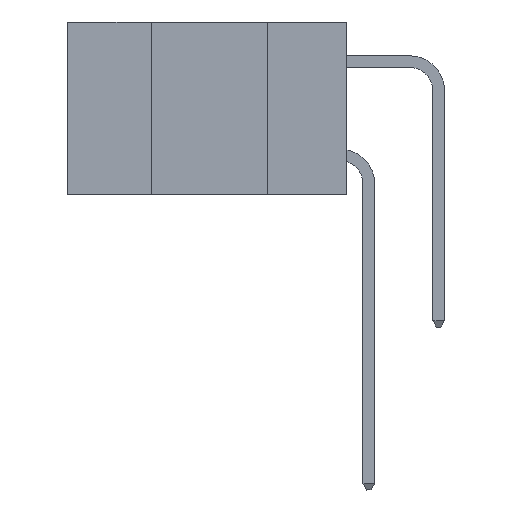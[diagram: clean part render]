
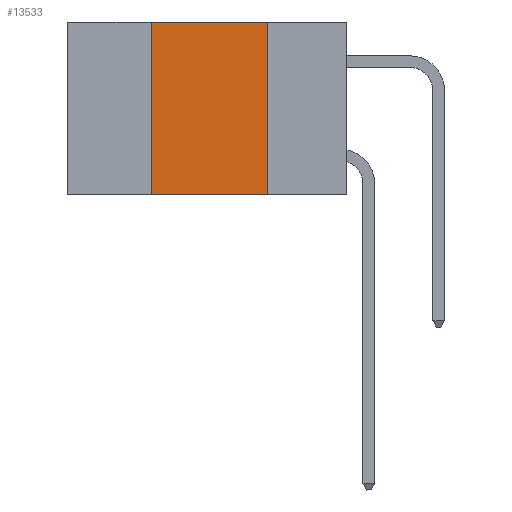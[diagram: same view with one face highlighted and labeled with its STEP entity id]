
A CAD part, left-side view. The second image highlights one B-rep face of the part: STEP entity #13533.
In plain terms, the highlighted planar face has unit normal (-1, 0, 0).
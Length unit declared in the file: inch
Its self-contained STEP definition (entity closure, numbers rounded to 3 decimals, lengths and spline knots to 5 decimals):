
#81 = CARTESIAN_POINT ( 'NONE',  ( 0., 0.42, 0. ) ) ;
#253 = CARTESIAN_POINT ( 'NONE',  ( 0., 0.42, 0. ) ) ;
#668 = VECTOR ( 'NONE', #27522, 39.37008 ) ;
#1162 = ORIENTED_EDGE ( 'NONE', *, *, #27968, .T. ) ;
#1390 = CARTESIAN_POINT ( 'NONE',  ( 0., 0.6, 0. ) ) ;
#2509 = DIRECTION ( 'NONE',  ( 0., 0., 1. ) ) ;
#2756 = LINE ( 'NONE', #1390, #22796 ) ;
#3090 = PLANE ( 'NONE',  #19438 ) ;
#3829 = DIRECTION ( 'NONE',  ( 0., -1., 0. ) ) ;
#4033 = ORIENTED_EDGE ( 'NONE', *, *, #8613, .F. ) ;
#4258 = LINE ( 'NONE', #253, #22100 ) ;
#8543 = ORIENTED_EDGE ( 'NONE', *, *, #23736, .F. ) ;
#8613 = EDGE_CURVE ( 'NONE', #28833, #11055, #2756, .T. ) ;
#8774 = VERTEX_POINT ( 'NONE', #10993 ) ;
#10419 = DIRECTION ( 'NONE',  ( 0., 0., -1. ) ) ;
#10993 = CARTESIAN_POINT ( 'NONE',  ( 0., 0.17, -0.37 ) ) ;
#11025 = CARTESIAN_POINT ( 'NONE',  ( 0., 0.17, 0. ) ) ;
#11055 = VERTEX_POINT ( 'NONE', #11025 ) ;
#12737 = CARTESIAN_POINT ( 'NONE',  ( 0., 0.6, 0. ) ) ;
#13533 = ADVANCED_FACE ( 'NONE', ( #28286 ), #3090, .F. ) ;
#13978 = DIRECTION ( 'NONE',  ( 0., -1., 0. ) ) ;
#15574 = CARTESIAN_POINT ( 'NONE',  ( 0., 0.17, 0. ) ) ;
#15886 = VECTOR ( 'NONE', #13978, 39.37008 ) ;
#15972 = LINE ( 'NONE', #15574, #668 ) ;
#19438 = AXIS2_PLACEMENT_3D ( 'NONE', #12737, #19555, #10419 ) ;
#19555 = DIRECTION ( 'NONE',  ( 1., 0., 0. ) ) ;
#22086 = LINE ( 'NONE', #25537, #15886 ) ;
#22100 = VECTOR ( 'NONE', #2509, 39.37008 ) ;
#22796 = VECTOR ( 'NONE', #3829, 39.37008 ) ;
#23736 = EDGE_CURVE ( 'NONE', #24186, #28833, #4258, .T. ) ;
#24186 = VERTEX_POINT ( 'NONE', #25321 ) ;
#25321 = CARTESIAN_POINT ( 'NONE',  ( 0., 0.42, -0.37 ) ) ;
#25537 = CARTESIAN_POINT ( 'NONE',  ( 0., 0.6, -0.37 ) ) ;
#26533 = EDGE_CURVE ( 'NONE', #11055, #8774, #15972, .T. ) ;
#27522 = DIRECTION ( 'NONE',  ( 0., 0., -1. ) ) ;
#27968 = EDGE_CURVE ( 'NONE', #24186, #8774, #22086, .T. ) ;
#28286 = FACE_OUTER_BOUND ( 'NONE', #29885, .T. ) ;
#28833 = VERTEX_POINT ( 'NONE', #81 ) ;
#29431 = ORIENTED_EDGE ( 'NONE', *, *, #26533, .F. ) ;
#29885 = EDGE_LOOP ( 'NONE', ( #29431, #4033, #8543, #1162 ) ) ;
